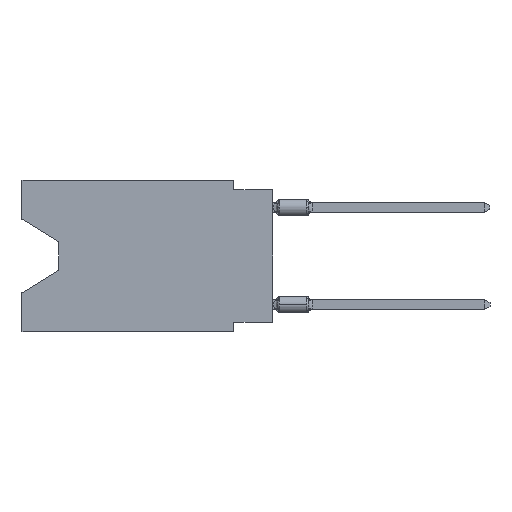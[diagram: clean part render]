
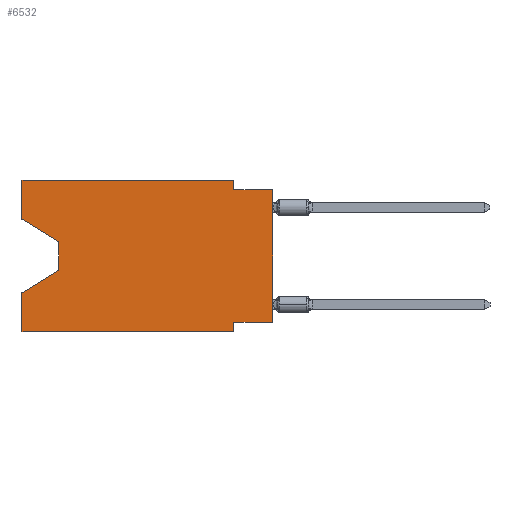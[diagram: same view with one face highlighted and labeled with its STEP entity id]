
A CAD part, left-side view. The second image highlights one B-rep face of the part: STEP entity #6532.
In plain terms, the highlighted planar face has unit normal (-1, 0, 0).
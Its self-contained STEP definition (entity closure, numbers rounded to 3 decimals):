
#35 = VECTOR ( 'NONE', #22673, 1000. ) ;
#215 = CARTESIAN_POINT ( 'NONE',  ( 0., 16.383, -2.546 ) ) ;
#424 = EDGE_CURVE ( 'NONE', #22015, #21315, #9860, .T. ) ;
#704 = EDGE_CURVE ( 'NONE', #7365, #21315, #4722, .T. ) ;
#882 = VECTOR ( 'NONE', #22203, 1000. ) ;
#938 = CARTESIAN_POINT ( 'NONE',  ( 0., 0., -9.271 ) ) ;
#1021 = DIRECTION ( 'NONE',  ( 0., 0., 1. ) ) ;
#1375 = VERTEX_POINT ( 'NONE', #215 ) ;
#1400 = DIRECTION ( 'NONE',  ( 0., 0., -1. ) ) ;
#1598 = ORIENTED_EDGE ( 'NONE', *, *, #8741, .F. ) ;
#1668 = EDGE_CURVE ( 'NONE', #22183, #22498, #13661, .T. ) ;
#2062 = DIRECTION ( 'NONE',  ( 0., 0., -1. ) ) ;
#2196 = EDGE_CURVE ( 'NONE', #16412, #22498, #12367, .T. ) ;
#2269 = LINE ( 'NONE', #9287, #17841 ) ;
#2322 = DIRECTION ( 'NONE',  ( 0., 0., -1. ) ) ;
#2454 = CARTESIAN_POINT ( 'NONE',  ( 0., 2.54, -0.635 ) ) ;
#2593 = CARTESIAN_POINT ( 'NONE',  ( 0., 16.383, 0. ) ) ;
#2905 = LINE ( 'NONE', #15254, #3517 ) ;
#3190 = LINE ( 'NONE', #20825, #11240 ) ;
#3517 = VECTOR ( 'NONE', #9933, 1000. ) ;
#4630 = CARTESIAN_POINT ( 'NONE',  ( 0., 16.383, -9.906 ) ) ;
#4691 = CARTESIAN_POINT ( 'NONE',  ( 0., 13.97, -5.893 ) ) ;
#4722 = LINE ( 'NONE', #15232, #15618 ) ;
#5043 = ORIENTED_EDGE ( 'NONE', *, *, #7420, .T. ) ;
#5544 = ORIENTED_EDGE ( 'NONE', *, *, #10630, .F. ) ;
#6229 = CARTESIAN_POINT ( 'NONE',  ( 0., 2.54, 0. ) ) ;
#6305 = ORIENTED_EDGE ( 'NONE', *, *, #704, .F. ) ;
#6320 = EDGE_CURVE ( 'NONE', #22015, #22152, #2905, .T. ) ;
#6532 = ADVANCED_FACE ( 'NONE', ( #10621 ), #6592, .F. ) ;
#6592 = PLANE ( 'NONE',  #19754 ) ;
#6779 = ORIENTED_EDGE ( 'NONE', *, *, #13427, .T. ) ;
#7365 = VERTEX_POINT ( 'NONE', #13560 ) ;
#7420 = EDGE_CURVE ( 'NONE', #18302, #22152, #10109, .T. ) ;
#7947 = DIRECTION ( 'NONE',  ( 0., 1., 0. ) ) ;
#8121 = CARTESIAN_POINT ( 'NONE',  ( 0., 16.383, -9.906 ) ) ;
#8317 = VECTOR ( 'NONE', #22573, 1000. ) ;
#8396 = CARTESIAN_POINT ( 'NONE',  ( 0., 0., -0.635 ) ) ;
#8488 = VECTOR ( 'NONE', #17694, 1000. ) ;
#8741 = EDGE_CURVE ( 'NONE', #1375, #20298, #20393, .T. ) ;
#9077 = CARTESIAN_POINT ( 'NONE',  ( 0., 13.97, -4.013 ) ) ;
#9287 = CARTESIAN_POINT ( 'NONE',  ( 0., 16.383, -2.546 ) ) ;
#9860 = LINE ( 'NONE', #8121, #882 ) ;
#9933 = DIRECTION ( 'NONE',  ( 0., 0., 1. ) ) ;
#10109 = LINE ( 'NONE', #4691, #8317 ) ;
#10134 = ORIENTED_EDGE ( 'NONE', *, *, #11731, .F. ) ;
#10480 = CARTESIAN_POINT ( 'NONE',  ( 0., 13.97, -5.893 ) ) ;
#10621 = FACE_OUTER_BOUND ( 'NONE', #20895, .T. ) ;
#10630 = EDGE_CURVE ( 'NONE', #15562, #16412, #18624, .T. ) ;
#10650 = VECTOR ( 'NONE', #1021, 1000. ) ;
#10697 = LINE ( 'NONE', #19594, #11595 ) ;
#11240 = VECTOR ( 'NONE', #12056, 1000. ) ;
#11446 = CARTESIAN_POINT ( 'NONE',  ( 0., 2.54, 0. ) ) ;
#11595 = VECTOR ( 'NONE', #2062, 1000. ) ;
#11731 = EDGE_CURVE ( 'NONE', #20298, #15562, #3190, .T. ) ;
#12056 = DIRECTION ( 'NONE',  ( 0., -1., 0. ) ) ;
#12367 = LINE ( 'NONE', #12476, #8488 ) ;
#12476 = CARTESIAN_POINT ( 'NONE',  ( 0., 0., -0.635 ) ) ;
#13142 = LINE ( 'NONE', #938, #19823 ) ;
#13427 = EDGE_CURVE ( 'NONE', #1375, #19790, #2269, .T. ) ;
#13560 = CARTESIAN_POINT ( 'NONE',  ( 0., 2.54, -9.271 ) ) ;
#13619 = CARTESIAN_POINT ( 'NONE',  ( 0., 16.383, 0. ) ) ;
#13661 = LINE ( 'NONE', #20705, #35 ) ;
#14888 = VECTOR ( 'NONE', #22302, 1000. ) ;
#15232 = CARTESIAN_POINT ( 'NONE',  ( 0., 2.54, -9.906 ) ) ;
#15254 = CARTESIAN_POINT ( 'NONE',  ( 0., 16.383, 0. ) ) ;
#15291 = ORIENTED_EDGE ( 'NONE', *, *, #6320, .F. ) ;
#15328 = CARTESIAN_POINT ( 'NONE',  ( 0., 16.383, 0. ) ) ;
#15330 = ORIENTED_EDGE ( 'NONE', *, *, #19794, .T. ) ;
#15368 = CARTESIAN_POINT ( 'NONE',  ( 0., 16.383, -7.36 ) ) ;
#15488 = CARTESIAN_POINT ( 'NONE',  ( 0., 0., -9.271 ) ) ;
#15529 = EDGE_CURVE ( 'NONE', #22183, #7365, #13142, .T. ) ;
#15562 = VERTEX_POINT ( 'NONE', #6229 ) ;
#15618 = VECTOR ( 'NONE', #1400, 1000. ) ;
#16412 = VERTEX_POINT ( 'NONE', #2454 ) ;
#17571 = ORIENTED_EDGE ( 'NONE', *, *, #424, .T. ) ;
#17618 = CARTESIAN_POINT ( 'NONE',  ( 0., 2.54, -9.906 ) ) ;
#17694 = DIRECTION ( 'NONE',  ( 0., -1., 0. ) ) ;
#17841 = VECTOR ( 'NONE', #19688, 1000. ) ;
#18228 = ORIENTED_EDGE ( 'NONE', *, *, #2196, .F. ) ;
#18302 = VERTEX_POINT ( 'NONE', #10480 ) ;
#18624 = LINE ( 'NONE', #11446, #14888 ) ;
#19594 = CARTESIAN_POINT ( 'NONE',  ( 0., 13.97, -4.013 ) ) ;
#19688 = DIRECTION ( 'NONE',  ( 0., -0.855, -0.519 ) ) ;
#19754 = AXIS2_PLACEMENT_3D ( 'NONE', #13619, #20667, #2322 ) ;
#19790 = VERTEX_POINT ( 'NONE', #9077 ) ;
#19794 = EDGE_CURVE ( 'NONE', #19790, #18302, #10697, .T. ) ;
#19823 = VECTOR ( 'NONE', #7947, 1000. ) ;
#20298 = VERTEX_POINT ( 'NONE', #2593 ) ;
#20393 = LINE ( 'NONE', #15328, #10650 ) ;
#20646 = ORIENTED_EDGE ( 'NONE', *, *, #1668, .T. ) ;
#20667 = DIRECTION ( 'NONE',  ( 1., 0., 0. ) ) ;
#20705 = CARTESIAN_POINT ( 'NONE',  ( 0., 0., 0. ) ) ;
#20825 = CARTESIAN_POINT ( 'NONE',  ( 0., 16.383, 0. ) ) ;
#20895 = EDGE_LOOP ( 'NONE', ( #6779, #15330, #5043, #15291, #17571, #6305, #22705, #20646, #18228, #5544, #10134, #1598 ) ) ;
#21315 = VERTEX_POINT ( 'NONE', #17618 ) ;
#22015 = VERTEX_POINT ( 'NONE', #4630 ) ;
#22152 = VERTEX_POINT ( 'NONE', #15368 ) ;
#22183 = VERTEX_POINT ( 'NONE', #15488 ) ;
#22203 = DIRECTION ( 'NONE',  ( 0., -1., 0. ) ) ;
#22302 = DIRECTION ( 'NONE',  ( 0., 0., -1. ) ) ;
#22498 = VERTEX_POINT ( 'NONE', #8396 ) ;
#22573 = DIRECTION ( 'NONE',  ( 0., 0.855, -0.519 ) ) ;
#22673 = DIRECTION ( 'NONE',  ( 0., 0., 1. ) ) ;
#22705 = ORIENTED_EDGE ( 'NONE', *, *, #15529, .F. ) ;
